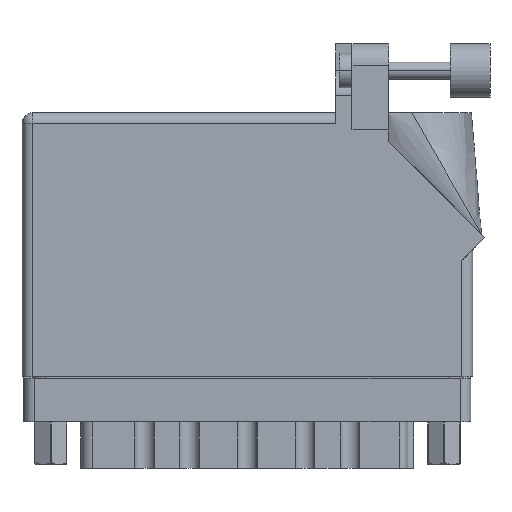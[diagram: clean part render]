
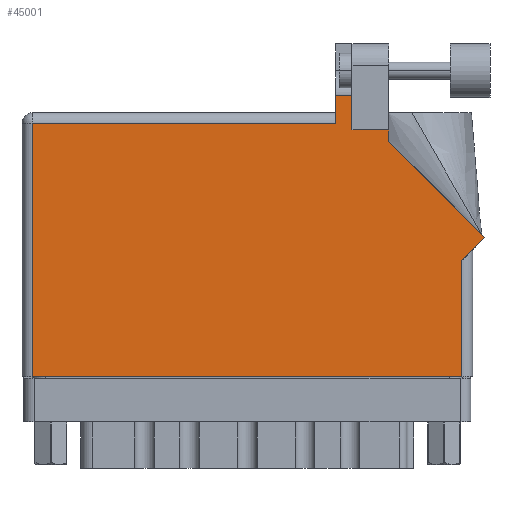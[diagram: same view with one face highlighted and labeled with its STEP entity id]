
A CAD part, front view. The second image highlights one B-rep face of the part: STEP entity #45001.
In plain terms, the highlighted face is planar.
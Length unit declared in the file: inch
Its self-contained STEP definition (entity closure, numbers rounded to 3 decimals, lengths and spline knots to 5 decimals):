
#169 = LINE ( 'NONE', #24019, #22088 ) ;
#494 = CARTESIAN_POINT ( 'NONE',  ( 0.062, 0., 0. ) ) ;
#885 = LINE ( 'NONE', #59919, #44750 ) ;
#1338 = CARTESIAN_POINT ( 'NONE',  ( 2.55, 0.737, 0. ) ) ;
#1623 = VECTOR ( 'NONE', #31158, 39.37008 ) ;
#2004 = VERTEX_POINT ( 'NONE', #40401 ) ;
#2037 = EDGE_CURVE ( 'NONE', #28354, #23788, #29666, .T. ) ;
#2408 = AXIS2_PLACEMENT_3D ( 'NONE', #4343, #52323, #57586 ) ;
#2753 = EDGE_CURVE ( 'NONE', #9334, #55771, #29097, .T. ) ;
#3923 = PLANE ( 'NONE',  #2408 ) ;
#4138 = DIRECTION ( 'NONE',  ( 0., -1., 0. ) ) ;
#4236 = ORIENTED_EDGE ( 'NONE', *, *, #2753, .T. ) ;
#4343 = CARTESIAN_POINT ( 'NONE',  ( 0., 1.53, 0. ) ) ;
#4648 = CARTESIAN_POINT ( 'NONE',  ( 0.062, 1.468, 0. ) ) ;
#4930 = ORIENTED_EDGE ( 'NONE', *, *, #60585, .T. ) ;
#5672 = CARTESIAN_POINT ( 'NONE',  ( 1.819, 1.6315, 0. ) ) ;
#5987 = EDGE_CURVE ( 'NONE', #62640, #59634, #30728, .T. ) ;
#8277 = CARTESIAN_POINT ( 'NONE',  ( 1.913, 1.6315, 0. ) ) ;
#8546 = ORIENTED_EDGE ( 'NONE', *, *, #12950, .T. ) ;
#9334 = VERTEX_POINT ( 'NONE', #23849 ) ;
#10434 = EDGE_CURVE ( 'NONE', #39685, #2004, #33985, .T. ) ;
#10942 = VERTEX_POINT ( 'NONE', #60605 ) ;
#12674 = CARTESIAN_POINT ( 'NONE',  ( 0., 0., 0. ) ) ;
#12950 = EDGE_CURVE ( 'NONE', #55771, #28354, #62550, .T. ) ;
#13718 = CARTESIAN_POINT ( 'NONE',  ( 2.24377, 1.6315, 0. ) ) ;
#15783 = CARTESIAN_POINT ( 'NONE',  ( 2.55, 0., 0. ) ) ;
#16111 = EDGE_LOOP ( 'NONE', ( #57031, #31606, #47741, #38747, #48818, #4236, #8546, #41058, #24194, #24924, #4930 ) ) ;
#16158 = CARTESIAN_POINT ( 'NONE',  ( 2.68271, 0.80771, 0. ) ) ;
#16691 = EDGE_CURVE ( 'NONE', #10942, #41343, #885, .T. ) ;
#17392 = VECTOR ( 'NONE', #24902, 39.37008 ) ;
#17418 = FACE_OUTER_BOUND ( 'NONE', #16111, .T. ) ;
#17701 = CARTESIAN_POINT ( 'NONE',  ( 2.68271, 0.80771, 0. ) ) ;
#18764 = DIRECTION ( 'NONE',  ( -0.707, 0.707, 0. ) ) ;
#21158 = DIRECTION ( 'NONE',  ( 0., 1., 0. ) ) ;
#21417 = LINE ( 'NONE', #494, #39542 ) ;
#22088 = VECTOR ( 'NONE', #4138, 39.37008 ) ;
#23788 = VERTEX_POINT ( 'NONE', #16158 ) ;
#23849 = CARTESIAN_POINT ( 'NONE',  ( 0.062, 0., 0. ) ) ;
#24019 = CARTESIAN_POINT ( 'NONE',  ( 1.819, 1.53, 0. ) ) ;
#24194 = ORIENTED_EDGE ( 'NONE', *, *, #36220, .T. ) ;
#24902 = DIRECTION ( 'NONE',  ( -1., 0., 0. ) ) ;
#24924 = ORIENTED_EDGE ( 'NONE', *, *, #10434, .T. ) ;
#28078 = VECTOR ( 'NONE', #18764, 39.37008 ) ;
#28354 = VERTEX_POINT ( 'NONE', #32446 ) ;
#29097 = LINE ( 'NONE', #12674, #56289 ) ;
#29666 = LINE ( 'NONE', #53964, #38752 ) ;
#29907 = DIRECTION ( 'NONE',  ( 0., 1., 0. ) ) ;
#30511 = EDGE_CURVE ( 'NONE', #59634, #9334, #21417, .T. ) ;
#30728 = LINE ( 'NONE', #58694, #17392 ) ;
#31138 = DIRECTION ( 'NONE',  ( 0.707, 0.707, 0. ) ) ;
#31158 = DIRECTION ( 'NONE',  ( -1., 0., 0. ) ) ;
#31355 = CARTESIAN_POINT ( 'NONE',  ( 2.126, 1.43, 0. ) ) ;
#31606 = ORIENTED_EDGE ( 'NONE', *, *, #40201, .T. ) ;
#32446 = CARTESIAN_POINT ( 'NONE',  ( 2.55, 0.675, 0. ) ) ;
#32928 = DIRECTION ( 'NONE',  ( -1., 0., 0. ) ) ;
#33985 = LINE ( 'NONE', #45891, #61998 ) ;
#34304 = DIRECTION ( 'NONE',  ( 0., -1., 0. ) ) ;
#36220 = EDGE_CURVE ( 'NONE', #23788, #39685, #41629, .T. ) ;
#37072 = VECTOR ( 'NONE', #32928, 39.37008 ) ;
#38747 = ORIENTED_EDGE ( 'NONE', *, *, #5987, .T. ) ;
#38752 = VECTOR ( 'NONE', #31138, 39.37008 ) ;
#39542 = VECTOR ( 'NONE', #34304, 39.37008 ) ;
#39685 = VERTEX_POINT ( 'NONE', #52255 ) ;
#40201 = EDGE_CURVE ( 'NONE', #41343, #42198, #53988, .T. ) ;
#40401 = CARTESIAN_POINT ( 'NONE',  ( 2.126, 1.43, 0. ) ) ;
#41058 = ORIENTED_EDGE ( 'NONE', *, *, #2037, .T. ) ;
#41343 = VERTEX_POINT ( 'NONE', #8277 ) ;
#41601 = DIRECTION ( 'NONE',  ( 1., 0., 0. ) ) ;
#41629 = LINE ( 'NONE', #17701, #28078 ) ;
#42198 = VERTEX_POINT ( 'NONE', #5672 ) ;
#43961 = LINE ( 'NONE', #31355, #1623 ) ;
#44425 = EDGE_CURVE ( 'NONE', #42198, #62640, #169, .T. ) ;
#44750 = VECTOR ( 'NONE', #60549, 39.37008 ) ;
#45001 = ADVANCED_FACE ( 'NONE', ( #17418 ), #3923, .F. ) ;
#45891 = CARTESIAN_POINT ( 'NONE',  ( 2.126, 1.36442, 0. ) ) ;
#47741 = ORIENTED_EDGE ( 'NONE', *, *, #44425, .T. ) ;
#48818 = ORIENTED_EDGE ( 'NONE', *, *, #30511, .T. ) ;
#52199 = CARTESIAN_POINT ( 'NONE',  ( 1.819, 1.468, 0. ) ) ;
#52255 = CARTESIAN_POINT ( 'NONE',  ( 2.126, 1.36442, 0. ) ) ;
#52323 = DIRECTION ( 'NONE',  ( 0., 0., -1. ) ) ;
#53964 = CARTESIAN_POINT ( 'NONE',  ( 2.612, 0.737, 0. ) ) ;
#53988 = LINE ( 'NONE', #13718, #37072 ) ;
#55771 = VERTEX_POINT ( 'NONE', #15783 ) ;
#56289 = VECTOR ( 'NONE', #41601, 39.37008 ) ;
#56501 = VECTOR ( 'NONE', #29907, 39.37008 ) ;
#57031 = ORIENTED_EDGE ( 'NONE', *, *, #16691, .T. ) ;
#57586 = DIRECTION ( 'NONE',  ( -1., 0., 0. ) ) ;
#58694 = CARTESIAN_POINT ( 'NONE',  ( 0., 1.468, 0. ) ) ;
#59634 = VERTEX_POINT ( 'NONE', #4648 ) ;
#59919 = CARTESIAN_POINT ( 'NONE',  ( 1.913, 1.43, 0. ) ) ;
#60549 = DIRECTION ( 'NONE',  ( 0., 1., 0. ) ) ;
#60585 = EDGE_CURVE ( 'NONE', #2004, #10942, #43961, .T. ) ;
#60605 = CARTESIAN_POINT ( 'NONE',  ( 1.913, 1.43, 0. ) ) ;
#61998 = VECTOR ( 'NONE', #21158, 39.37008 ) ;
#62550 = LINE ( 'NONE', #1338, #56501 ) ;
#62640 = VERTEX_POINT ( 'NONE', #52199 ) ;
